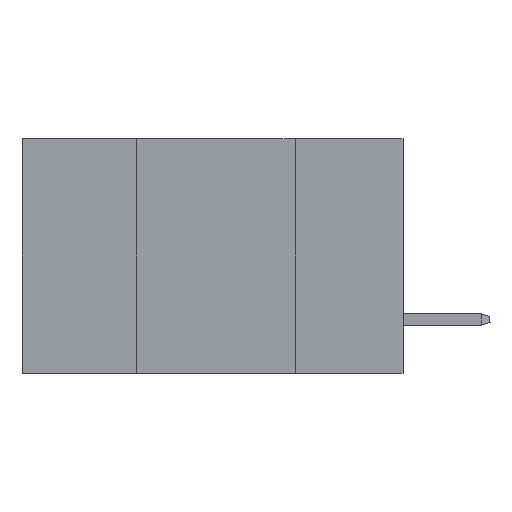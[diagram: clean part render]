
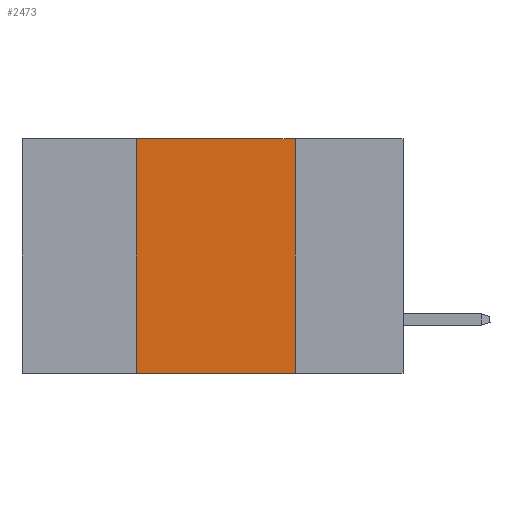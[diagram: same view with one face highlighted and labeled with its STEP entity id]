
A CAD part, left-side view. The second image highlights one B-rep face of the part: STEP entity #2473.
In plain terms, the highlighted planar face has unit normal (-1, 0, 0).
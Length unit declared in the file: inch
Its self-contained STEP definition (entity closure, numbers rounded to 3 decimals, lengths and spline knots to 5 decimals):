
#75 = VERTEX_POINT ( 'NONE', #3841 ) ;
#481 = CARTESIAN_POINT ( 'NONE',  ( 0., 0.17, -0.37 ) ) ;
#583 = VERTEX_POINT ( 'NONE', #13901 ) ;
#870 = DIRECTION ( 'NONE',  ( 0., -1., 0. ) ) ;
#1063 = VECTOR ( 'NONE', #8214, 39.37008 ) ;
#1630 = DIRECTION ( 'NONE',  ( 1., 0., 0. ) ) ;
#1681 = DIRECTION ( 'NONE',  ( 0., -1., 0. ) ) ;
#2361 = CARTESIAN_POINT ( 'NONE',  ( 0., 0.17, 0. ) ) ;
#2473 = ADVANCED_FACE ( 'NONE', ( #18054 ), #17948, .F. ) ;
#3432 = CARTESIAN_POINT ( 'NONE',  ( 0., 0.42, -0.37 ) ) ;
#3641 = VERTEX_POINT ( 'NONE', #481 ) ;
#3841 = CARTESIAN_POINT ( 'NONE',  ( 0., 0.42, 0. ) ) ;
#4944 = DIRECTION ( 'NONE',  ( 0., 0., -1. ) ) ;
#6099 = VERTEX_POINT ( 'NONE', #3432 ) ;
#6369 = LINE ( 'NONE', #16210, #1063 ) ;
#6889 = ORIENTED_EDGE ( 'NONE', *, *, #11598, .F. ) ;
#7235 = VECTOR ( 'NONE', #870, 39.37008 ) ;
#7326 = CARTESIAN_POINT ( 'NONE',  ( 0., 0.6, -0.37 ) ) ;
#7987 = CARTESIAN_POINT ( 'NONE',  ( 0., 0.6, 0. ) ) ;
#8214 = DIRECTION ( 'NONE',  ( 0., 0., 1. ) ) ;
#9967 = VECTOR ( 'NONE', #1681, 39.37008 ) ;
#11598 = EDGE_CURVE ( 'NONE', #6099, #75, #6369, .T. ) ;
#11866 = AXIS2_PLACEMENT_3D ( 'NONE', #7987, #1630, #4944 ) ;
#12469 = ORIENTED_EDGE ( 'NONE', *, *, #19794, .F. ) ;
#12771 = CARTESIAN_POINT ( 'NONE',  ( 0., 0.6, 0. ) ) ;
#13569 = EDGE_CURVE ( 'NONE', #6099, #3641, #15632, .T. ) ;
#13901 = CARTESIAN_POINT ( 'NONE',  ( 0., 0.17, 0. ) ) ;
#14204 = DIRECTION ( 'NONE',  ( 0., 0., -1. ) ) ;
#15053 = ORIENTED_EDGE ( 'NONE', *, *, #19427, .F. ) ;
#15245 = ORIENTED_EDGE ( 'NONE', *, *, #13569, .T. ) ;
#15632 = LINE ( 'NONE', #7326, #7235 ) ;
#16210 = CARTESIAN_POINT ( 'NONE',  ( 0., 0.42, 0. ) ) ;
#17948 = PLANE ( 'NONE',  #11866 ) ;
#18054 = FACE_OUTER_BOUND ( 'NONE', #18069, .T. ) ;
#18069 = EDGE_LOOP ( 'NONE', ( #15053, #12469, #6889, #15245 ) ) ;
#18876 = LINE ( 'NONE', #2361, #18915 ) ;
#18915 = VECTOR ( 'NONE', #14204, 39.37008 ) ;
#19259 = LINE ( 'NONE', #12771, #9967 ) ;
#19427 = EDGE_CURVE ( 'NONE', #583, #3641, #18876, .T. ) ;
#19794 = EDGE_CURVE ( 'NONE', #75, #583, #19259, .T. ) ;
